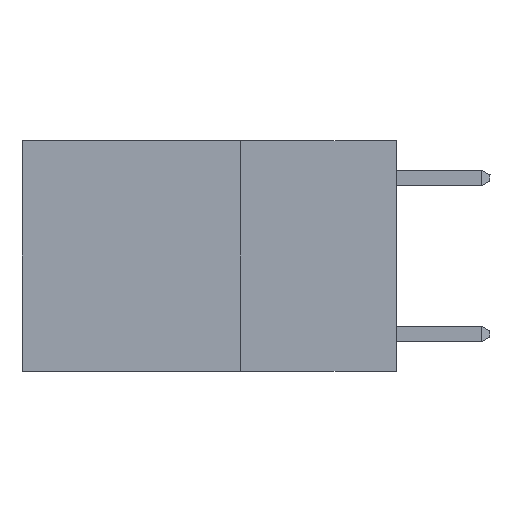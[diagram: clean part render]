
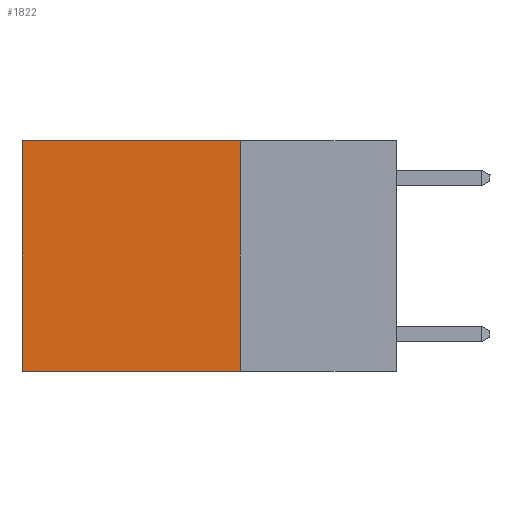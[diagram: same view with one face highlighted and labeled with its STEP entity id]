
A CAD part, left-side view. The second image highlights one B-rep face of the part: STEP entity #1822.
In plain terms, the highlighted planar face has unit normal (-1, 0, 0).
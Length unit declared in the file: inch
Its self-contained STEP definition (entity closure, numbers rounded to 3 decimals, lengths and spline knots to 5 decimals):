
#114 = DIRECTION ( 'NONE',  ( 0., 0., -1. ) ) ;
#690 = VECTOR ( 'NONE', #6867, 39.37008 ) ;
#1172 = VERTEX_POINT ( 'NONE', #15991 ) ;
#1270 = CARTESIAN_POINT ( 'NONE',  ( 0.2625, 0.25, -0.37 ) ) ;
#1822 = ADVANCED_FACE ( 'NONE', ( #14565 ), #16134, .F. ) ;
#1958 = LINE ( 'NONE', #19928, #690 ) ;
#4449 = LINE ( 'NONE', #17816, #10196 ) ;
#6387 = VERTEX_POINT ( 'NONE', #11134 ) ;
#6594 = DIRECTION ( 'NONE',  ( 0., 1., 0. ) ) ;
#6867 = DIRECTION ( 'NONE',  ( 0., 0., -1. ) ) ;
#7552 = VECTOR ( 'NONE', #114, 39.37008 ) ;
#7624 = EDGE_CURVE ( 'NONE', #6387, #1172, #1958, .T. ) ;
#9152 = ORIENTED_EDGE ( 'NONE', *, *, #13393, .F. ) ;
#9674 = CARTESIAN_POINT ( 'NONE',  ( 0.2625, 0.25, 0. ) ) ;
#10196 = VECTOR ( 'NONE', #6594, 39.37008 ) ;
#11134 = CARTESIAN_POINT ( 'NONE',  ( 0.2625, 0.6, 0. ) ) ;
#12430 = DIRECTION ( 'NONE',  ( 1., 0., 0. ) ) ;
#13035 = CARTESIAN_POINT ( 'NONE',  ( 0.2625, 0.25, 0. ) ) ;
#13244 = LINE ( 'NONE', #13035, #22381 ) ;
#13266 = LINE ( 'NONE', #13712, #7552 ) ;
#13393 = EDGE_CURVE ( 'NONE', #18269, #1172, #4449, .T. ) ;
#13471 = AXIS2_PLACEMENT_3D ( 'NONE', #19679, #12430, #19767 ) ;
#13712 = CARTESIAN_POINT ( 'NONE',  ( 0.2625, 0.25, 0. ) ) ;
#14182 = ORIENTED_EDGE ( 'NONE', *, *, #20693, .F. ) ;
#14508 = VERTEX_POINT ( 'NONE', #9674 ) ;
#14565 = FACE_OUTER_BOUND ( 'NONE', #14896, .T. ) ;
#14896 = EDGE_LOOP ( 'NONE', ( #16563, #9152, #14182, #17205 ) ) ;
#14903 = DIRECTION ( 'NONE',  ( 0., 1., 0. ) ) ;
#15991 = CARTESIAN_POINT ( 'NONE',  ( 0.2625, 0.6, -0.37 ) ) ;
#16134 = PLANE ( 'NONE',  #13471 ) ;
#16563 = ORIENTED_EDGE ( 'NONE', *, *, #7624, .T. ) ;
#17205 = ORIENTED_EDGE ( 'NONE', *, *, #21164, .T. ) ;
#17816 = CARTESIAN_POINT ( 'NONE',  ( 0.2625, 0.25, -0.37 ) ) ;
#18269 = VERTEX_POINT ( 'NONE', #1270 ) ;
#19679 = CARTESIAN_POINT ( 'NONE',  ( 0.2625, 0.25, 0. ) ) ;
#19767 = DIRECTION ( 'NONE',  ( 0., 0., -1. ) ) ;
#19928 = CARTESIAN_POINT ( 'NONE',  ( 0.2625, 0.6, 0. ) ) ;
#20693 = EDGE_CURVE ( 'NONE', #14508, #18269, #13266, .T. ) ;
#21164 = EDGE_CURVE ( 'NONE', #14508, #6387, #13244, .T. ) ;
#22381 = VECTOR ( 'NONE', #14903, 39.37008 ) ;
